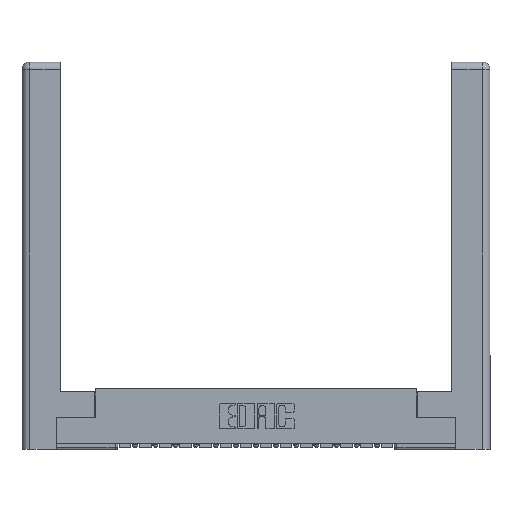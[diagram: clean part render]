
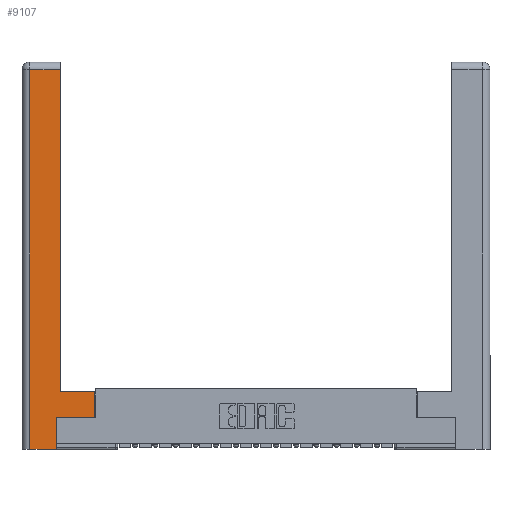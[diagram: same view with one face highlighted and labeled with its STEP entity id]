
A CAD part, top view. The second image highlights one B-rep face of the part: STEP entity #9107.
In plain terms, the highlighted planar face has unit normal (0, 0, 1).
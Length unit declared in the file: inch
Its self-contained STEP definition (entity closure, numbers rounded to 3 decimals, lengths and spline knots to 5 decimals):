
#305 = VERTEX_POINT ( 'NONE', #18245 ) ;
#338 = DIRECTION ( 'NONE',  ( -1., 0., 0. ) ) ;
#410 = EDGE_CURVE ( 'NONE', #8544, #305, #5130, .T. ) ;
#510 = ORIENTED_EDGE ( 'NONE', *, *, #410, .T. ) ;
#730 = CARTESIAN_POINT ( 'NONE',  ( 0.565, 0.45, 0. ) ) ;
#747 = CARTESIAN_POINT ( 'NONE',  ( 0.565, 0.45, 0. ) ) ;
#1070 = CARTESIAN_POINT ( 'NONE',  ( 0.295, 0.45, 0. ) ) ;
#1095 = CARTESIAN_POINT ( 'NONE',  ( 0.0615, 2.94, 0. ) ) ;
#1194 = LINE ( 'NONE', #1095, #2237 ) ;
#1332 = EDGE_CURVE ( 'NONE', #5560, #4574, #1194, .T. ) ;
#1943 = EDGE_CURVE ( 'NONE', #3648, #8544, #2409, .T. ) ;
#2237 = VECTOR ( 'NONE', #15965, 39.37008 ) ;
#2258 = DIRECTION ( 'NONE',  ( 1., 0., 0. ) ) ;
#2367 = VERTEX_POINT ( 'NONE', #747 ) ;
#2409 = LINE ( 'NONE', #16976, #5339 ) ;
#2499 = CARTESIAN_POINT ( 'NONE',  ( 0.0615, 2.94, 0. ) ) ;
#2793 = EDGE_LOOP ( 'NONE', ( #8473, #6417, #7018, #16042, #14415, #510, #17864, #9074 ) ) ;
#2843 = CARTESIAN_POINT ( 'NONE',  ( 0.295, 3., 0. ) ) ;
#3416 = DIRECTION ( 'NONE',  ( 0., 1., 0. ) ) ;
#3449 = CARTESIAN_POINT ( 'NONE',  ( 0.295, 2.94, 0. ) ) ;
#3615 = EDGE_CURVE ( 'NONE', #6524, #3648, #12478, .T. ) ;
#3648 = VERTEX_POINT ( 'NONE', #11506 ) ;
#4574 = VERTEX_POINT ( 'NONE', #2499 ) ;
#4625 = DIRECTION ( 'NONE',  ( 0., -1., 0. ) ) ;
#5130 = LINE ( 'NONE', #9674, #7389 ) ;
#5339 = VECTOR ( 'NONE', #15428, 39.37008 ) ;
#5408 = DIRECTION ( 'NONE',  ( -1., 0., 0. ) ) ;
#5560 = VERTEX_POINT ( 'NONE', #3449 ) ;
#5885 = VECTOR ( 'NONE', #2258, 39.37008 ) ;
#6142 = PLANE ( 'NONE',  #17825 ) ;
#6417 = ORIENTED_EDGE ( 'NONE', *, *, #1332, .T. ) ;
#6524 = VERTEX_POINT ( 'NONE', #15642 ) ;
#7018 = ORIENTED_EDGE ( 'NONE', *, *, #13459, .T. ) ;
#7389 = VECTOR ( 'NONE', #8308, 39.37008 ) ;
#7515 = VERTEX_POINT ( 'NONE', #8359 ) ;
#7783 = DIRECTION ( 'NONE',  ( 0., 0., -1. ) ) ;
#7984 = EDGE_CURVE ( 'NONE', #305, #2367, #15481, .T. ) ;
#8308 = DIRECTION ( 'NONE',  ( 1., 0., 0. ) ) ;
#8359 = CARTESIAN_POINT ( 'NONE',  ( 0.295, 0.45, 0. ) ) ;
#8473 = ORIENTED_EDGE ( 'NONE', *, *, #18846, .T. ) ;
#8544 = VERTEX_POINT ( 'NONE', #10425 ) ;
#9074 = ORIENTED_EDGE ( 'NONE', *, *, #11555, .T. ) ;
#9107 = ADVANCED_FACE ( 'NONE', ( #13675 ), #6142, .F. ) ;
#9663 = VECTOR ( 'NONE', #13257, 39.37008 ) ;
#9674 = CARTESIAN_POINT ( 'NONE',  ( 0.565, 0.245, 0. ) ) ;
#10425 = CARTESIAN_POINT ( 'NONE',  ( 0.265, 0.245, 0. ) ) ;
#11506 = CARTESIAN_POINT ( 'NONE',  ( 0.265, 0., 0. ) ) ;
#11555 = EDGE_CURVE ( 'NONE', #2367, #7515, #15933, .T. ) ;
#11669 = LINE ( 'NONE', #17567, #17918 ) ;
#11995 = VECTOR ( 'NONE', #5408, 39.37008 ) ;
#12478 = LINE ( 'NONE', #15462, #5885 ) ;
#13162 = VECTOR ( 'NONE', #3416, 39.37008 ) ;
#13257 = DIRECTION ( 'NONE',  ( 0., 1., 0. ) ) ;
#13459 = EDGE_CURVE ( 'NONE', #4574, #6524, #11669, .T. ) ;
#13675 = FACE_OUTER_BOUND ( 'NONE', #2793, .T. ) ;
#14415 = ORIENTED_EDGE ( 'NONE', *, *, #1943, .T. ) ;
#14906 = LINE ( 'NONE', #2843, #9663 ) ;
#15428 = DIRECTION ( 'NONE',  ( 0., 1., 0. ) ) ;
#15462 = CARTESIAN_POINT ( 'NONE',  ( 0.265, 0., 0. ) ) ;
#15481 = LINE ( 'NONE', #730, #13162 ) ;
#15642 = CARTESIAN_POINT ( 'NONE',  ( 0.0615, 0., 0. ) ) ;
#15933 = LINE ( 'NONE', #1070, #11995 ) ;
#15965 = DIRECTION ( 'NONE',  ( -1., 0., 0. ) ) ;
#16042 = ORIENTED_EDGE ( 'NONE', *, *, #3615, .T. ) ;
#16381 = CARTESIAN_POINT ( 'NONE',  ( 0., 0., 0. ) ) ;
#16976 = CARTESIAN_POINT ( 'NONE',  ( 0.265, 0.245, 0. ) ) ;
#17567 = CARTESIAN_POINT ( 'NONE',  ( 0.0615, 0., 0. ) ) ;
#17825 = AXIS2_PLACEMENT_3D ( 'NONE', #16381, #7783, #338 ) ;
#17864 = ORIENTED_EDGE ( 'NONE', *, *, #7984, .T. ) ;
#17918 = VECTOR ( 'NONE', #4625, 39.37008 ) ;
#18245 = CARTESIAN_POINT ( 'NONE',  ( 0.565, 0.245, 0. ) ) ;
#18846 = EDGE_CURVE ( 'NONE', #7515, #5560, #14906, .T. ) ;
